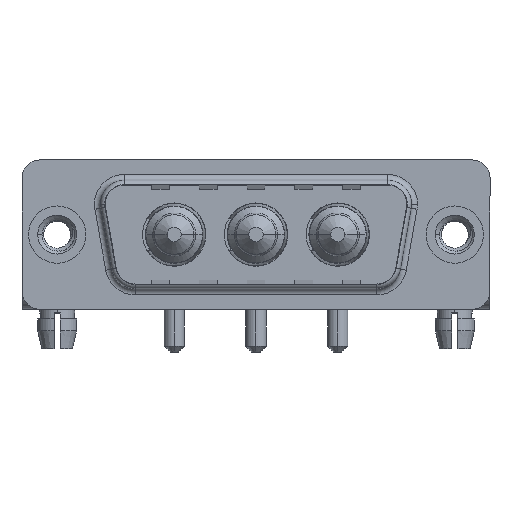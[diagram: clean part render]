
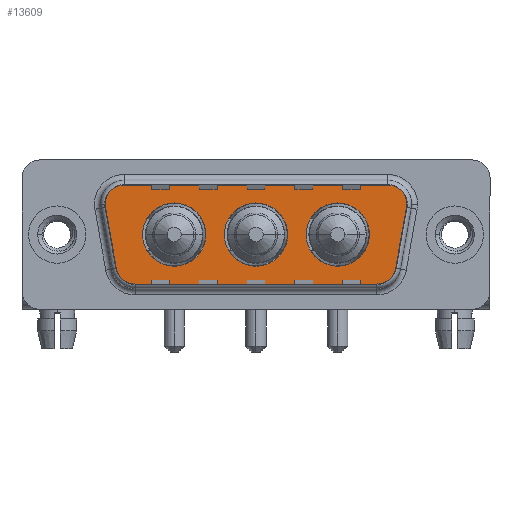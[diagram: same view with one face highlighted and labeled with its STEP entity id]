
A CAD part, top view. The second image highlights one B-rep face of the part: STEP entity #13609.
In plain terms, the highlighted planar face has unit normal (0, 0, 1).
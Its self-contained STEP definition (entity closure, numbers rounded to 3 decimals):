
#4 = VERTEX_POINT ( 'NONE', #9115 ) ;
#73 = LINE ( 'NONE', #6202, #11677 ) ;
#568 = DIRECTION ( 'NONE',  ( 1., 0., 0. ) ) ;
#627 = DIRECTION ( 'NONE',  ( 1., 0., 0. ) ) ;
#637 = CIRCLE ( 'NONE', #11263, 2. ) ;
#1077 = VERTEX_POINT ( 'NONE', #6403 ) ;
#1489 = LINE ( 'NONE', #6153, #7592 ) ;
#1654 = CIRCLE ( 'NONE', #14732, 2. ) ;
#1860 = CIRCLE ( 'NONE', #3092, 2.65 ) ;
#1873 = PLANE ( 'NONE',  #12466 ) ;
#1976 = CARTESIAN_POINT ( 'NONE',  ( 5.411, 4.9, 0. ) ) ;
#2030 = DIRECTION ( 'NONE',  ( 0., 0., 1. ) ) ;
#2040 = AXIS2_PLACEMENT_3D ( 'NONE', #11409, #13940, #5537 ) ;
#2210 = CARTESIAN_POINT ( 'NONE',  ( 27.889, 4.9, 0. ) ) ;
#2265 = LINE ( 'NONE', #6849, #6044 ) ;
#2339 = VERTEX_POINT ( 'NONE', #9553 ) ;
#2627 = CIRCLE ( 'NONE', #15194, 2.65 ) ;
#2643 = AXIS2_PLACEMENT_3D ( 'NONE', #13552, #6623, #13476 ) ;
#2723 = DIRECTION ( 'NONE',  ( 0., 0., 1. ) ) ;
#2795 = CARTESIAN_POINT ( 'NONE',  ( 23.5, 0., 0. ) ) ;
#2834 = EDGE_CURVE ( 'NONE', #4, #7886, #1860, .T. ) ;
#2882 = CARTESIAN_POINT ( 'NONE',  ( 27.889, 2.9, 0. ) ) ;
#3092 = AXIS2_PLACEMENT_3D ( 'NONE', #14018, #3437, #10615 ) ;
#3258 = AXIS2_PLACEMENT_3D ( 'NONE', #3494, #13154, #8522 ) ;
#3421 = CARTESIAN_POINT ( 'NONE',  ( 26.866, -2.9, 0. ) ) ;
#3437 = DIRECTION ( 'NONE',  ( 0., 0., 1. ) ) ;
#3494 = CARTESIAN_POINT ( 'NONE',  ( 5.411, 2.9, 0. ) ) ;
#3506 = CARTESIAN_POINT ( 'NONE',  ( 26.866, -4.9, 0. ) ) ;
#3734 = CARTESIAN_POINT ( 'NONE',  ( 29.859, 2.553, 0. ) ) ;
#3831 = DIRECTION ( 'NONE',  ( 0.174, 0.985, 0. ) ) ;
#4021 = VERTEX_POINT ( 'NONE', #2210 ) ;
#4078 = ORIENTED_EDGE ( 'NONE', *, *, #2834, .F. ) ;
#4160 = VERTEX_POINT ( 'NONE', #5692 ) ;
#4529 = EDGE_CURVE ( 'NONE', #12214, #13537, #5116, .T. ) ;
#4613 = VERTEX_POINT ( 'NONE', #3506 ) ;
#4841 = ORIENTED_EDGE ( 'NONE', *, *, #6504, .T. ) ;
#5116 = CIRCLE ( 'NONE', #2643, 2.65 ) ;
#5511 = FACE_BOUND ( 'NONE', #12905, .T. ) ;
#5537 = DIRECTION ( 'NONE',  ( -1., 0., 0. ) ) ;
#5692 = CARTESIAN_POINT ( 'NONE',  ( 5.411, 4.9, 0. ) ) ;
#5841 = EDGE_CURVE ( 'NONE', #4021, #4160, #15025, .T. ) ;
#6044 = VECTOR ( 'NONE', #12789, 1000. ) ;
#6078 = EDGE_CURVE ( 'NONE', #8785, #10116, #1489, .T. ) ;
#6153 = CARTESIAN_POINT ( 'NONE',  ( 29.859, 2.553, 0. ) ) ;
#6202 = CARTESIAN_POINT ( 'NONE',  ( 3.441, 2.553, 0. ) ) ;
#6403 = CARTESIAN_POINT ( 'NONE',  ( 4.464, -3.247, 0. ) ) ;
#6428 = CARTESIAN_POINT ( 'NONE',  ( 28.836, -3.247, 0. ) ) ;
#6504 = EDGE_CURVE ( 'NONE', #4613, #8785, #1654, .T. ) ;
#6607 = DIRECTION ( 'NONE',  ( 0., 0., 1. ) ) ;
#6623 = DIRECTION ( 'NONE',  ( 0., 0., 1. ) ) ;
#6849 = CARTESIAN_POINT ( 'NONE',  ( 6.434, -4.9, 0. ) ) ;
#6908 = CARTESIAN_POINT ( 'NONE',  ( 12.45, 0., 0. ) ) ;
#6961 = VERTEX_POINT ( 'NONE', #13567 ) ;
#7453 = CIRCLE ( 'NONE', #3258, 2. ) ;
#7463 = ORIENTED_EDGE ( 'NONE', *, *, #5841, .T. ) ;
#7519 = ORIENTED_EDGE ( 'NONE', *, *, #13529, .T. ) ;
#7592 = VECTOR ( 'NONE', #3831, 1000. ) ;
#7832 = ORIENTED_EDGE ( 'NONE', *, *, #4529, .F. ) ;
#7886 = VERTEX_POINT ( 'NONE', #13108 ) ;
#7978 = EDGE_LOOP ( 'NONE', ( #7832, #11340 ) ) ;
#8186 = DIRECTION ( 'NONE',  ( 0., 0., 1. ) ) ;
#8309 = EDGE_CURVE ( 'NONE', #7886, #4, #8629, .T. ) ;
#8522 = DIRECTION ( 'NONE',  ( 1., 0., 0. ) ) ;
#8570 = EDGE_CURVE ( 'NONE', #6961, #10013, #10095, .T. ) ;
#8593 = ORIENTED_EDGE ( 'NONE', *, *, #14979, .T. ) ;
#8629 = CIRCLE ( 'NONE', #9592, 2.65 ) ;
#8785 = VERTEX_POINT ( 'NONE', #6428 ) ;
#8908 = DIRECTION ( 'NONE',  ( -1., 0., 0. ) ) ;
#8981 = DIRECTION ( 'NONE',  ( 0., 0., 1. ) ) ;
#9061 = FACE_BOUND ( 'NONE', #7978, .T. ) ;
#9071 = ORIENTED_EDGE ( 'NONE', *, *, #8570, .F. ) ;
#9115 = CARTESIAN_POINT ( 'NONE',  ( 26.15, 0., 0. ) ) ;
#9286 = DIRECTION ( 'NONE',  ( 0., 0., 1. ) ) ;
#9350 = DIRECTION ( 'NONE',  ( 0.174, -0.985, 0. ) ) ;
#9475 = EDGE_CURVE ( 'NONE', #14315, #4021, #12891, .T. ) ;
#9550 = ORIENTED_EDGE ( 'NONE', *, *, #8309, .F. ) ;
#9553 = CARTESIAN_POINT ( 'NONE',  ( 6.434, -4.9, 0. ) ) ;
#9591 = DIRECTION ( 'NONE',  ( 1., 0., 0. ) ) ;
#9592 = AXIS2_PLACEMENT_3D ( 'NONE', #2795, #2723, #11064 ) ;
#9636 = CARTESIAN_POINT ( 'NONE',  ( 19.3, 0., 0. ) ) ;
#9789 = VECTOR ( 'NONE', #11330, 1000. ) ;
#9892 = ORIENTED_EDGE ( 'NONE', *, *, #10140, .T. ) ;
#10013 = VERTEX_POINT ( 'NONE', #6908 ) ;
#10037 = ORIENTED_EDGE ( 'NONE', *, *, #11769, .T. ) ;
#10062 = DIRECTION ( 'NONE',  ( 1., 0., 0. ) ) ;
#10095 = CIRCLE ( 'NONE', #13312, 2.65 ) ;
#10116 = VERTEX_POINT ( 'NONE', #3734 ) ;
#10140 = EDGE_CURVE ( 'NONE', #4160, #13335, #7453, .T. ) ;
#10369 = DIRECTION ( 'NONE',  ( -1., 0., 0. ) ) ;
#10518 = CARTESIAN_POINT ( 'NONE',  ( 6.434, -2.9, 0. ) ) ;
#10615 = DIRECTION ( 'NONE',  ( 1., 0., 0. ) ) ;
#10654 = DIRECTION ( 'NONE',  ( 1., 0., 0. ) ) ;
#11064 = DIRECTION ( 'NONE',  ( 1., 0., 0. ) ) ;
#11095 = DIRECTION ( 'NONE',  ( 0., 0., 1. ) ) ;
#11223 = CARTESIAN_POINT ( 'NONE',  ( 26.866, -2.9, 0. ) ) ;
#11263 = AXIS2_PLACEMENT_3D ( 'NONE', #10518, #9286, #10369 ) ;
#11330 = DIRECTION ( 'NONE',  ( -1., 0., 0. ) ) ;
#11340 = ORIENTED_EDGE ( 'NONE', *, *, #14207, .F. ) ;
#11386 = FACE_BOUND ( 'NONE', #12455, .T. ) ;
#11409 = CARTESIAN_POINT ( 'NONE',  ( 27.889, 2.9, 0. ) ) ;
#11598 = CARTESIAN_POINT ( 'NONE',  ( 9.8, 0., 0. ) ) ;
#11677 = VECTOR ( 'NONE', #9350, 1000. ) ;
#11769 = EDGE_CURVE ( 'NONE', #13335, #1077, #73, .T. ) ;
#12214 = VERTEX_POINT ( 'NONE', #9636 ) ;
#12380 = CARTESIAN_POINT ( 'NONE',  ( 14., 0., 0. ) ) ;
#12455 = EDGE_LOOP ( 'NONE', ( #15281, #9071 ) ) ;
#12462 = FACE_OUTER_BOUND ( 'NONE', #13408, .T. ) ;
#12466 = AXIS2_PLACEMENT_3D ( 'NONE', #11223, #6607, #627 ) ;
#12624 = CARTESIAN_POINT ( 'NONE',  ( 9.8, 0., 0. ) ) ;
#12742 = CIRCLE ( 'NONE', #14456, 2.65 ) ;
#12789 = DIRECTION ( 'NONE',  ( 1., 0., 0. ) ) ;
#12891 = CIRCLE ( 'NONE', #2040, 2. ) ;
#12905 = EDGE_LOOP ( 'NONE', ( #4078, #9550 ) ) ;
#13108 = CARTESIAN_POINT ( 'NONE',  ( 20.85, 0., 0. ) ) ;
#13154 = DIRECTION ( 'NONE',  ( 0., 0., 1. ) ) ;
#13257 = EDGE_CURVE ( 'NONE', #2339, #4613, #2265, .T. ) ;
#13302 = DIRECTION ( 'NONE',  ( 0., 0., 1. ) ) ;
#13312 = AXIS2_PLACEMENT_3D ( 'NONE', #11598, #8186, #10654 ) ;
#13314 = CARTESIAN_POINT ( 'NONE',  ( 3.441, 2.553, 0. ) ) ;
#13335 = VERTEX_POINT ( 'NONE', #13314 ) ;
#13408 = EDGE_LOOP ( 'NONE', ( #4841, #14274, #7519, #14915, #7463, #9892, #10037, #8593, #13684 ) ) ;
#13476 = DIRECTION ( 'NONE',  ( 1., 0., 0. ) ) ;
#13529 = EDGE_CURVE ( 'NONE', #10116, #14315, #14927, .T. ) ;
#13537 = VERTEX_POINT ( 'NONE', #12380 ) ;
#13552 = CARTESIAN_POINT ( 'NONE',  ( 16.65, 0., 0. ) ) ;
#13567 = CARTESIAN_POINT ( 'NONE',  ( 7.15, 0., 0. ) ) ;
#13609 = ADVANCED_FACE ( 'NONE', ( #9061, #5511, #11386, #12462 ), #1873, .T. ) ;
#13684 = ORIENTED_EDGE ( 'NONE', *, *, #13257, .T. ) ;
#13940 = DIRECTION ( 'NONE',  ( 0., 0., 1. ) ) ;
#14018 = CARTESIAN_POINT ( 'NONE',  ( 23.5, 0., 0. ) ) ;
#14207 = EDGE_CURVE ( 'NONE', #13537, #12214, #12742, .T. ) ;
#14274 = ORIENTED_EDGE ( 'NONE', *, *, #6078, .T. ) ;
#14315 = VERTEX_POINT ( 'NONE', #15089 ) ;
#14456 = AXIS2_PLACEMENT_3D ( 'NONE', #14714, #11095, #568 ) ;
#14714 = CARTESIAN_POINT ( 'NONE',  ( 16.65, 0., 0. ) ) ;
#14732 = AXIS2_PLACEMENT_3D ( 'NONE', #3421, #13302, #9591 ) ;
#14796 = EDGE_CURVE ( 'NONE', #10013, #6961, #2627, .T. ) ;
#14915 = ORIENTED_EDGE ( 'NONE', *, *, #9475, .T. ) ;
#14927 = CIRCLE ( 'NONE', #15161, 2. ) ;
#14979 = EDGE_CURVE ( 'NONE', #1077, #2339, #637, .T. ) ;
#15025 = LINE ( 'NONE', #1976, #9789 ) ;
#15089 = CARTESIAN_POINT ( 'NONE',  ( 29.889, 2.9, 0. ) ) ;
#15161 = AXIS2_PLACEMENT_3D ( 'NONE', #2882, #8981, #8908 ) ;
#15194 = AXIS2_PLACEMENT_3D ( 'NONE', #12624, #2030, #10062 ) ;
#15281 = ORIENTED_EDGE ( 'NONE', *, *, #14796, .F. ) ;
